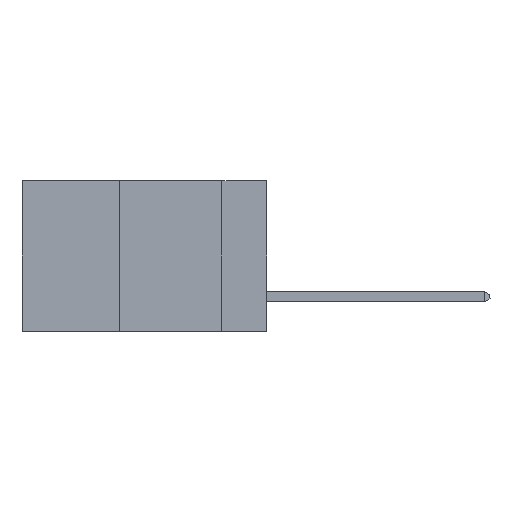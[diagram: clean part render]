
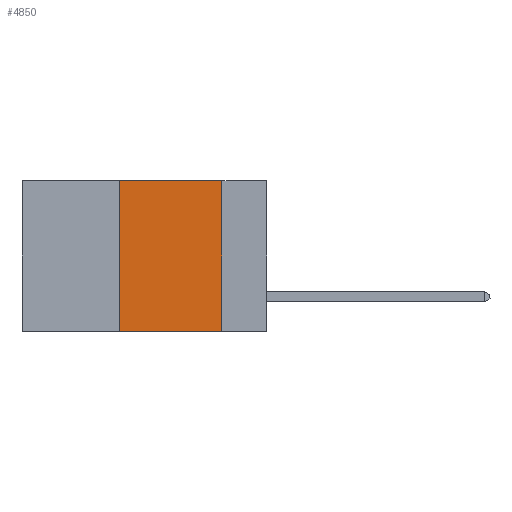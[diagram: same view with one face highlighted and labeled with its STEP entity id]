
A CAD part, left-side view. The second image highlights one B-rep face of the part: STEP entity #4850.
In plain terms, the highlighted planar face has unit normal (-1, 0, 0).
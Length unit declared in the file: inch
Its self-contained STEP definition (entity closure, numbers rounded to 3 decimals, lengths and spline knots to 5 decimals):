
#206 = LINE ( 'NONE', #623, #8260 ) ;
#240 = AXIS2_PLACEMENT_3D ( 'NONE', #264, #9435, #3182 ) ;
#264 = CARTESIAN_POINT ( 'NONE',  ( 0., 0.6, 0. ) ) ;
#509 = VECTOR ( 'NONE', #9626, 39.37008 ) ;
#623 = CARTESIAN_POINT ( 'NONE',  ( 0., 0.36, 0. ) ) ;
#1506 = LINE ( 'NONE', #10654, #509 ) ;
#2094 = CARTESIAN_POINT ( 'NONE',  ( 0., 0.6, 0. ) ) ;
#2127 = PLANE ( 'NONE',  #240 ) ;
#2300 = FACE_OUTER_BOUND ( 'NONE', #8178, .T. ) ;
#3182 = DIRECTION ( 'NONE',  ( 0., 0., -1. ) ) ;
#4295 = EDGE_CURVE ( 'NONE', #12204, #8513, #1506, .T. ) ;
#4727 = EDGE_CURVE ( 'NONE', #5762, #8513, #11592, .T. ) ;
#4850 = ADVANCED_FACE ( 'NONE', ( #2300 ), #2127, .F. ) ;
#5762 = VERTEX_POINT ( 'NONE', #8660 ) ;
#5807 = LINE ( 'NONE', #2094, #8211 ) ;
#5958 = ORIENTED_EDGE ( 'NONE', *, *, #8411, .F. ) ;
#7141 = CARTESIAN_POINT ( 'NONE',  ( 0., 0.11, -0.37 ) ) ;
#7177 = CARTESIAN_POINT ( 'NONE',  ( 0., 0.11, 0. ) ) ;
#8007 = DIRECTION ( 'NONE',  ( 0., 0., 1. ) ) ;
#8178 = EDGE_LOOP ( 'NONE', ( #12803, #8746, #5958, #8276 ) ) ;
#8211 = VECTOR ( 'NONE', #11471, 39.37008 ) ;
#8260 = VECTOR ( 'NONE', #8007, 39.37008 ) ;
#8276 = ORIENTED_EDGE ( 'NONE', *, *, #4295, .T. ) ;
#8411 = EDGE_CURVE ( 'NONE', #12204, #11266, #206, .T. ) ;
#8513 = VERTEX_POINT ( 'NONE', #7141 ) ;
#8660 = CARTESIAN_POINT ( 'NONE',  ( 0., 0.11, 0. ) ) ;
#8746 = ORIENTED_EDGE ( 'NONE', *, *, #10248, .F. ) ;
#8862 = VECTOR ( 'NONE', #11282, 39.37008 ) ;
#9027 = CARTESIAN_POINT ( 'NONE',  ( 0., 0.36, 0. ) ) ;
#9435 = DIRECTION ( 'NONE',  ( 1., 0., 0. ) ) ;
#9510 = CARTESIAN_POINT ( 'NONE',  ( 0., 0.36, -0.37 ) ) ;
#9626 = DIRECTION ( 'NONE',  ( 0., -1., 0. ) ) ;
#10248 = EDGE_CURVE ( 'NONE', #11266, #5762, #5807, .T. ) ;
#10654 = CARTESIAN_POINT ( 'NONE',  ( 0., 0.6, -0.37 ) ) ;
#11266 = VERTEX_POINT ( 'NONE', #9027 ) ;
#11282 = DIRECTION ( 'NONE',  ( 0., 0., -1. ) ) ;
#11471 = DIRECTION ( 'NONE',  ( 0., -1., 0. ) ) ;
#11592 = LINE ( 'NONE', #7177, #8862 ) ;
#12204 = VERTEX_POINT ( 'NONE', #9510 ) ;
#12803 = ORIENTED_EDGE ( 'NONE', *, *, #4727, .F. ) ;
